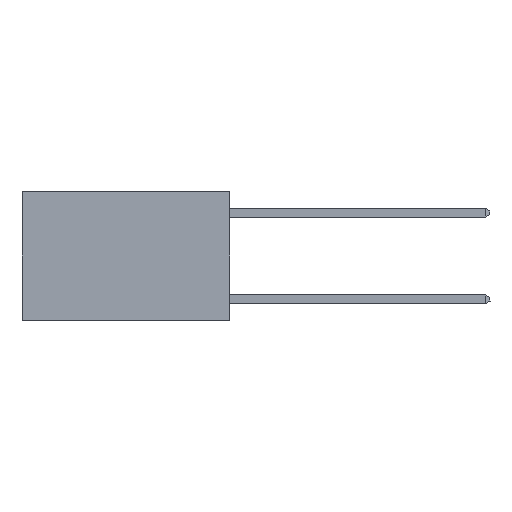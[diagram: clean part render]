
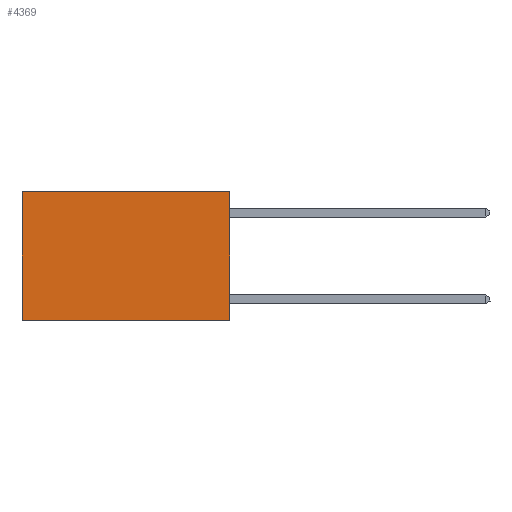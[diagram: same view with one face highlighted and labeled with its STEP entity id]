
A CAD part, left-side view. The second image highlights one B-rep face of the part: STEP entity #4369.
In plain terms, the highlighted planar face has unit normal (-1, 0, 0).
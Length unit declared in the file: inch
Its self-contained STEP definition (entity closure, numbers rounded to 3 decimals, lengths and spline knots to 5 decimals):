
#247 = DIRECTION ( 'NONE',  ( 0., 1., 0. ) ) ;
#1149 = VECTOR ( 'NONE', #8404, 39.37008 ) ;
#1634 = ORIENTED_EDGE ( 'NONE', *, *, #2669, .T. ) ;
#1729 = VERTEX_POINT ( 'NONE', #4514 ) ;
#1913 = LINE ( 'NONE', #6371, #10920 ) ;
#2190 = VERTEX_POINT ( 'NONE', #3257 ) ;
#2669 = EDGE_CURVE ( 'NONE', #1729, #2190, #3472, .T. ) ;
#3257 = CARTESIAN_POINT ( 'NONE',  ( 0.2625, 0.6, -0.37 ) ) ;
#3472 = LINE ( 'NONE', #10903, #1149 ) ;
#3696 = FACE_OUTER_BOUND ( 'NONE', #3850, .T. ) ;
#3763 = CARTESIAN_POINT ( 'NONE',  ( 0.2625, 0., 0. ) ) ;
#3850 = EDGE_LOOP ( 'NONE', ( #1634, #6458, #7651, #7813 ) ) ;
#4369 = ADVANCED_FACE ( 'NONE', ( #3696 ), #9946, .F. ) ;
#4514 = CARTESIAN_POINT ( 'NONE',  ( 0.2625, 0.6, 0. ) ) ;
#4571 = CARTESIAN_POINT ( 'NONE',  ( 0.2625, 0., 0. ) ) ;
#4664 = VECTOR ( 'NONE', #7237, 39.37008 ) ;
#4882 = DIRECTION ( 'NONE',  ( 0., 0., -1. ) ) ;
#5327 = EDGE_CURVE ( 'NONE', #6352, #9779, #10856, .T. ) ;
#5495 = CARTESIAN_POINT ( 'NONE',  ( 0.2625, 0., -0.37 ) ) ;
#6125 = CARTESIAN_POINT ( 'NONE',  ( 0.2625, 0., 0. ) ) ;
#6352 = VERTEX_POINT ( 'NONE', #4571 ) ;
#6371 = CARTESIAN_POINT ( 'NONE',  ( 0.2625, 0., -0.37 ) ) ;
#6458 = ORIENTED_EDGE ( 'NONE', *, *, #8241, .F. ) ;
#6851 = DIRECTION ( 'NONE',  ( 1., 0., 0. ) ) ;
#6965 = DIRECTION ( 'NONE',  ( 0., 0., -1. ) ) ;
#7035 = EDGE_CURVE ( 'NONE', #6352, #1729, #7277, .T. ) ;
#7237 = DIRECTION ( 'NONE',  ( 0., 1., 0. ) ) ;
#7277 = LINE ( 'NONE', #3763, #4664 ) ;
#7651 = ORIENTED_EDGE ( 'NONE', *, *, #5327, .F. ) ;
#7753 = CARTESIAN_POINT ( 'NONE',  ( 0.2625, 0., 0. ) ) ;
#7813 = ORIENTED_EDGE ( 'NONE', *, *, #7035, .T. ) ;
#7972 = AXIS2_PLACEMENT_3D ( 'NONE', #6125, #6851, #4882 ) ;
#8241 = EDGE_CURVE ( 'NONE', #9779, #2190, #1913, .T. ) ;
#8404 = DIRECTION ( 'NONE',  ( 0., 0., -1. ) ) ;
#8554 = VECTOR ( 'NONE', #6965, 39.37008 ) ;
#9779 = VERTEX_POINT ( 'NONE', #5495 ) ;
#9946 = PLANE ( 'NONE',  #7972 ) ;
#10856 = LINE ( 'NONE', #7753, #8554 ) ;
#10903 = CARTESIAN_POINT ( 'NONE',  ( 0.2625, 0.6, 0. ) ) ;
#10920 = VECTOR ( 'NONE', #247, 39.37008 ) ;
